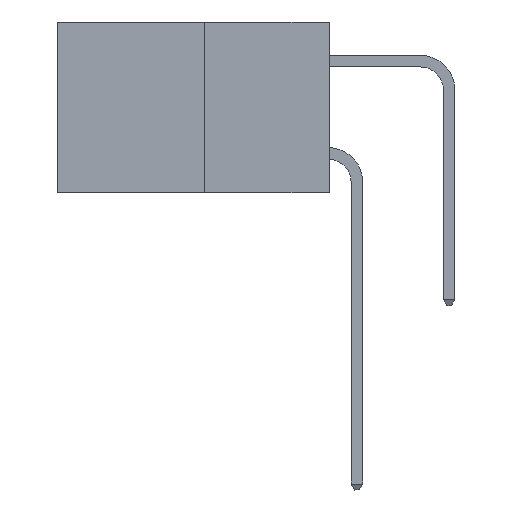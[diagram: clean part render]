
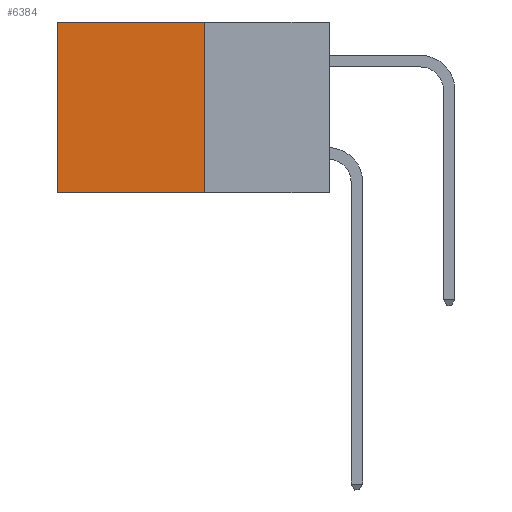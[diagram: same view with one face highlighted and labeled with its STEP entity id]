
A CAD part, left-side view. The second image highlights one B-rep face of the part: STEP entity #6384.
In plain terms, the highlighted planar face has unit normal (-1, 0, 0).
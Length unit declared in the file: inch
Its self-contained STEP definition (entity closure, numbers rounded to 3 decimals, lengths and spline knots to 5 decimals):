
#403 = CARTESIAN_POINT ( 'NONE',  ( 0.277, 0.27, -0.37 ) ) ;
#639 = ORIENTED_EDGE ( 'NONE', *, *, #15954, .F. ) ;
#795 = DIRECTION ( 'NONE',  ( 0., 0., -1. ) ) ;
#999 = LINE ( 'NONE', #2363, #10292 ) ;
#1128 = AXIS2_PLACEMENT_3D ( 'NONE', #11102, #7617, #7050 ) ;
#1599 = ORIENTED_EDGE ( 'NONE', *, *, #6506, .F. ) ;
#2153 = CARTESIAN_POINT ( 'NONE',  ( 0.277, 0.59, 0. ) ) ;
#2363 = CARTESIAN_POINT ( 'NONE',  ( 0.277, 0.27, -0.37 ) ) ;
#2433 = CARTESIAN_POINT ( 'NONE',  ( 0.277, 0.27, 0. ) ) ;
#2559 = EDGE_LOOP ( 'NONE', ( #15073, #639, #1599, #3124 ) ) ;
#3124 = ORIENTED_EDGE ( 'NONE', *, *, #15988, .T. ) ;
#3436 = PLANE ( 'NONE',  #1128 ) ;
#3613 = VERTEX_POINT ( 'NONE', #17301 ) ;
#3677 = VECTOR ( 'NONE', #8649, 39.37008 ) ;
#4476 = FACE_OUTER_BOUND ( 'NONE', #2559, .T. ) ;
#6384 = ADVANCED_FACE ( 'NONE', ( #4476 ), #3436, .F. ) ;
#6506 = EDGE_CURVE ( 'NONE', #3613, #9989, #7654, .T. ) ;
#7050 = DIRECTION ( 'NONE',  ( 0., 0., -1. ) ) ;
#7617 = DIRECTION ( 'NONE',  ( 1., 0., 0. ) ) ;
#7654 = LINE ( 'NONE', #403, #10331 ) ;
#8649 = DIRECTION ( 'NONE',  ( 0., 1., 0. ) ) ;
#9989 = VERTEX_POINT ( 'NONE', #17584 ) ;
#10292 = VECTOR ( 'NONE', #11726, 39.37008 ) ;
#10331 = VECTOR ( 'NONE', #795, 39.37008 ) ;
#11102 = CARTESIAN_POINT ( 'NONE',  ( 0.277, 0.27, -0.37 ) ) ;
#11726 = DIRECTION ( 'NONE',  ( 0., 1., 0. ) ) ;
#11837 = LINE ( 'NONE', #13962, #19080 ) ;
#12421 = VERTEX_POINT ( 'NONE', #13017 ) ;
#13017 = CARTESIAN_POINT ( 'NONE',  ( 0.277, 0.59, -0.37 ) ) ;
#13962 = CARTESIAN_POINT ( 'NONE',  ( 0.277, 0.59, -0.37 ) ) ;
#15073 = ORIENTED_EDGE ( 'NONE', *, *, #19253, .T. ) ;
#15801 = VERTEX_POINT ( 'NONE', #2153 ) ;
#15954 = EDGE_CURVE ( 'NONE', #9989, #12421, #999, .T. ) ;
#15988 = EDGE_CURVE ( 'NONE', #3613, #15801, #16619, .T. ) ;
#16619 = LINE ( 'NONE', #2433, #3677 ) ;
#17301 = CARTESIAN_POINT ( 'NONE',  ( 0.277, 0.27, 0. ) ) ;
#17584 = CARTESIAN_POINT ( 'NONE',  ( 0.277, 0.27, -0.37 ) ) ;
#19080 = VECTOR ( 'NONE', #20081, 39.37008 ) ;
#19253 = EDGE_CURVE ( 'NONE', #15801, #12421, #11837, .T. ) ;
#20081 = DIRECTION ( 'NONE',  ( 0., 0., -1. ) ) ;
